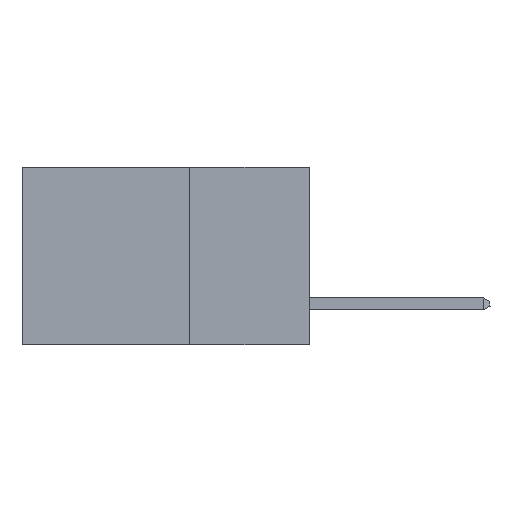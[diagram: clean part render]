
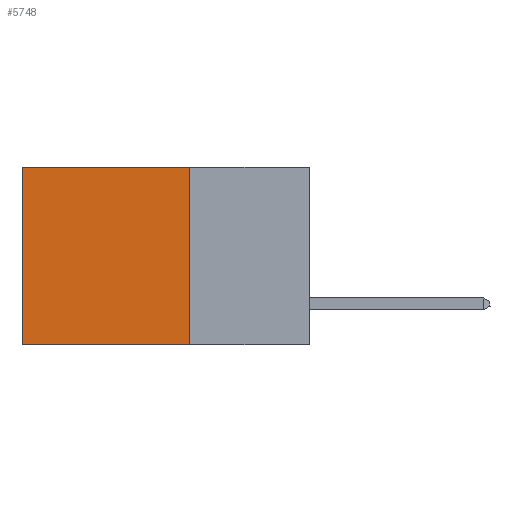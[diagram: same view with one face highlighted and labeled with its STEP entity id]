
A CAD part, left-side view. The second image highlights one B-rep face of the part: STEP entity #5748.
In plain terms, the highlighted planar face has unit normal (-1, 0, 0).
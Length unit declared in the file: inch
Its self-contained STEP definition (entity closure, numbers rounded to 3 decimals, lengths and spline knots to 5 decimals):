
#535 = FACE_OUTER_BOUND ( 'NONE', #4746, .T. ) ;
#1721 = CARTESIAN_POINT ( 'NONE',  ( 0.2875, 0.25, 0. ) ) ;
#4746 = EDGE_LOOP ( 'NONE', ( #30714, #15523, #12468, #43395 ) ) ;
#5748 = ADVANCED_FACE ( 'NONE', ( #535 ), #31843, .F. ) ;
#6666 = DIRECTION ( 'NONE',  ( 0., 0., -1. ) ) ;
#6936 = VERTEX_POINT ( 'NONE', #8684 ) ;
#7943 = VERTEX_POINT ( 'NONE', #43015 ) ;
#8684 = CARTESIAN_POINT ( 'NONE',  ( 0.2875, 0.6, -0.37 ) ) ;
#8691 = EDGE_CURVE ( 'NONE', #11200, #6936, #11947, .T. ) ;
#9273 = AXIS2_PLACEMENT_3D ( 'NONE', #28393, #42951, #25265 ) ;
#11200 = VERTEX_POINT ( 'NONE', #15429 ) ;
#11947 = LINE ( 'NONE', #21506, #34880 ) ;
#12468 = ORIENTED_EDGE ( 'NONE', *, *, #24070, .F. ) ;
#12920 = LINE ( 'NONE', #38458, #44848 ) ;
#14468 = DIRECTION ( 'NONE',  ( 0., 1., 0. ) ) ;
#15429 = CARTESIAN_POINT ( 'NONE',  ( 0.2875, 0.6, 0. ) ) ;
#15523 = ORIENTED_EDGE ( 'NONE', *, *, #28885, .F. ) ;
#17023 = DIRECTION ( 'NONE',  ( 0., 1., 0. ) ) ;
#21506 = CARTESIAN_POINT ( 'NONE',  ( 0.2875, 0.6, 0. ) ) ;
#22860 = CARTESIAN_POINT ( 'NONE',  ( 0.2875, 0.25, 0. ) ) ;
#24070 = EDGE_CURVE ( 'NONE', #38183, #7943, #44606, .T. ) ;
#25265 = DIRECTION ( 'NONE',  ( 0., 0., -1. ) ) ;
#28393 = CARTESIAN_POINT ( 'NONE',  ( 0.2875, 0.25, 0. ) ) ;
#28885 = EDGE_CURVE ( 'NONE', #7943, #6936, #39348, .T. ) ;
#29218 = VECTOR ( 'NONE', #14468, 39.37008 ) ;
#30714 = ORIENTED_EDGE ( 'NONE', *, *, #8691, .T. ) ;
#31843 = PLANE ( 'NONE',  #9273 ) ;
#33155 = DIRECTION ( 'NONE',  ( 0., 0., -1. ) ) ;
#34880 = VECTOR ( 'NONE', #6666, 39.37008 ) ;
#35744 = CARTESIAN_POINT ( 'NONE',  ( 0.2875, 0.25, -0.37 ) ) ;
#38183 = VERTEX_POINT ( 'NONE', #22860 ) ;
#38458 = CARTESIAN_POINT ( 'NONE',  ( 0.2875, 0.25, 0. ) ) ;
#38992 = VECTOR ( 'NONE', #33155, 39.37008 ) ;
#39348 = LINE ( 'NONE', #35744, #29218 ) ;
#41417 = EDGE_CURVE ( 'NONE', #38183, #11200, #12920, .T. ) ;
#42951 = DIRECTION ( 'NONE',  ( 1., 0., 0. ) ) ;
#43015 = CARTESIAN_POINT ( 'NONE',  ( 0.2875, 0.25, -0.37 ) ) ;
#43395 = ORIENTED_EDGE ( 'NONE', *, *, #41417, .T. ) ;
#44606 = LINE ( 'NONE', #1721, #38992 ) ;
#44848 = VECTOR ( 'NONE', #17023, 39.37008 ) ;
